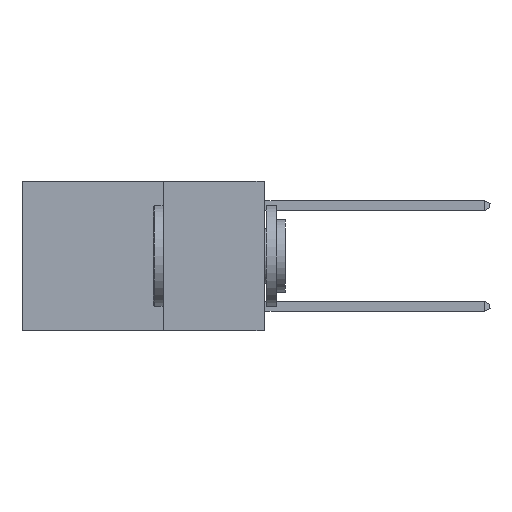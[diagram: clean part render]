
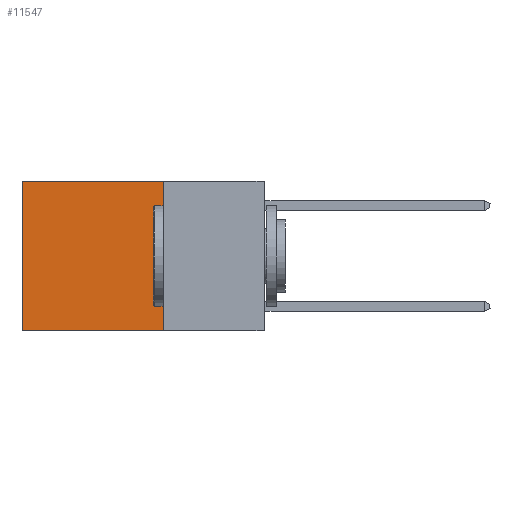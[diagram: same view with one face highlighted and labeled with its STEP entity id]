
A CAD part, left-side view. The second image highlights one B-rep face of the part: STEP entity #11547.
In plain terms, the highlighted planar face has unit normal (-1, 0, 0).
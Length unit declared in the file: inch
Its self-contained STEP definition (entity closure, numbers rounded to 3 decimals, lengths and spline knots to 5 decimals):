
#206 = EDGE_LOOP ( 'NONE', ( #13264, #11214, #21113, #22245 ) ) ;
#250 = VECTOR ( 'NONE', #25122, 39.37008 ) ;
#584 = VERTEX_POINT ( 'NONE', #25483 ) ;
#1689 = CARTESIAN_POINT ( 'NONE',  ( 0.2625, 0.25, 0. ) ) ;
#1816 = DIRECTION ( 'NONE',  ( 0., 0., -1. ) ) ;
#3278 = CARTESIAN_POINT ( 'NONE',  ( 0.2625, 0.25, -0.37 ) ) ;
#3306 = LINE ( 'NONE', #11525, #7196 ) ;
#4211 = LINE ( 'NONE', #12434, #9000 ) ;
#4727 = LINE ( 'NONE', #25666, #250 ) ;
#4885 = CARTESIAN_POINT ( 'NONE',  ( 0.2625, 0.25, 0. ) ) ;
#7055 = LINE ( 'NONE', #3278, #17607 ) ;
#7196 = VECTOR ( 'NONE', #25429, 39.37008 ) ;
#7914 = EDGE_CURVE ( 'NONE', #584, #23973, #3306, .T. ) ;
#8160 = PLANE ( 'NONE',  #22801 ) ;
#9000 = VECTOR ( 'NONE', #24599, 39.37008 ) ;
#9471 = VERTEX_POINT ( 'NONE', #23256 ) ;
#9494 = VERTEX_POINT ( 'NONE', #4885 ) ;
#9699 = EDGE_CURVE ( 'NONE', #9471, #23973, #7055, .T. ) ;
#10189 = FACE_OUTER_BOUND ( 'NONE', #206, .T. ) ;
#11214 = ORIENTED_EDGE ( 'NONE', *, *, #9699, .F. ) ;
#11525 = CARTESIAN_POINT ( 'NONE',  ( 0.2625, 0.6, 0. ) ) ;
#11547 = ADVANCED_FACE ( 'NONE', ( #10189 ), #8160, .F. ) ;
#12434 = CARTESIAN_POINT ( 'NONE',  ( 0.2625, 0.25, 0. ) ) ;
#13264 = ORIENTED_EDGE ( 'NONE', *, *, #7914, .T. ) ;
#17045 = EDGE_CURVE ( 'NONE', #9494, #9471, #4727, .T. ) ;
#17607 = VECTOR ( 'NONE', #19401, 39.37008 ) ;
#18063 = DIRECTION ( 'NONE',  ( 1., 0., 0. ) ) ;
#19401 = DIRECTION ( 'NONE',  ( 0., 1., 0. ) ) ;
#20367 = EDGE_CURVE ( 'NONE', #9494, #584, #4211, .T. ) ;
#21113 = ORIENTED_EDGE ( 'NONE', *, *, #17045, .F. ) ;
#22245 = ORIENTED_EDGE ( 'NONE', *, *, #20367, .T. ) ;
#22801 = AXIS2_PLACEMENT_3D ( 'NONE', #1689, #18063, #1816 ) ;
#23256 = CARTESIAN_POINT ( 'NONE',  ( 0.2625, 0.25, -0.37 ) ) ;
#23973 = VERTEX_POINT ( 'NONE', #25757 ) ;
#24599 = DIRECTION ( 'NONE',  ( 0., 1., 0. ) ) ;
#25122 = DIRECTION ( 'NONE',  ( 0., 0., -1. ) ) ;
#25429 = DIRECTION ( 'NONE',  ( 0., 0., -1. ) ) ;
#25483 = CARTESIAN_POINT ( 'NONE',  ( 0.2625, 0.6, 0. ) ) ;
#25666 = CARTESIAN_POINT ( 'NONE',  ( 0.2625, 0.25, 0. ) ) ;
#25757 = CARTESIAN_POINT ( 'NONE',  ( 0.2625, 0.6, -0.37 ) ) ;
